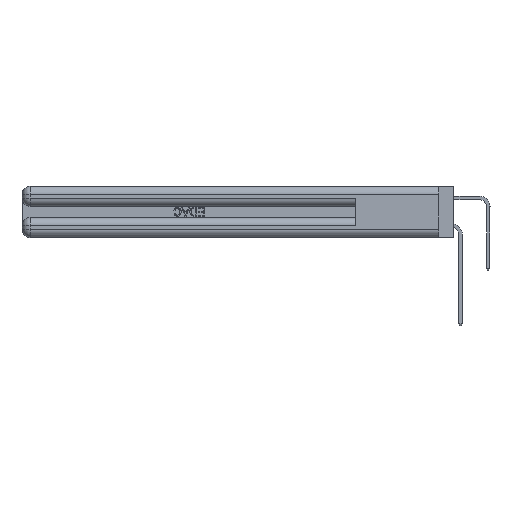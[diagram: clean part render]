
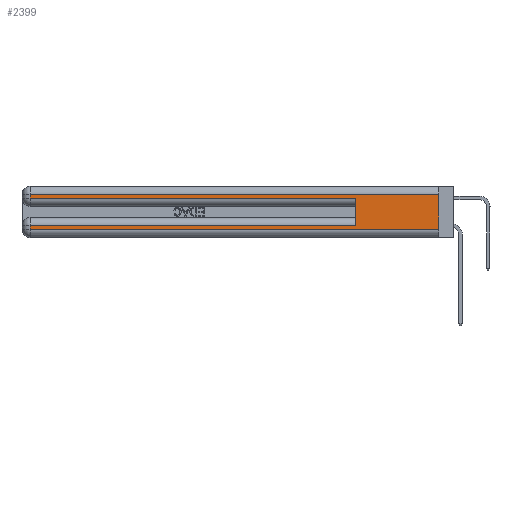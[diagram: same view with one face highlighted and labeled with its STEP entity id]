
A CAD part, left-side view. The second image highlights one B-rep face of the part: STEP entity #2399.
In plain terms, the highlighted planar face has unit normal (-1, 0, 0).
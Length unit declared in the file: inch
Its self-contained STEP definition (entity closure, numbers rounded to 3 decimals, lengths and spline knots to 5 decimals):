
#1094 = DIRECTION ( 'NONE',  ( 0., -1., 0. ) ) ;
#1205 = EDGE_CURVE ( 'NONE', #32645, #39011, #16985, .T. ) ;
#1219 = VECTOR ( 'NONE', #8162, 39.37008 ) ;
#2399 = ADVANCED_FACE ( 'NONE', ( #38661 ), #8370, .F. ) ;
#2451 = LINE ( 'NONE', #16035, #1219 ) ;
#2723 = VERTEX_POINT ( 'NONE', #14135 ) ;
#2846 = CARTESIAN_POINT ( 'NONE',  ( 0., 2.94, 0.085 ) ) ;
#3586 = LINE ( 'NONE', #7741, #32290 ) ;
#4106 = ORIENTED_EDGE ( 'NONE', *, *, #9121, .T. ) ;
#4197 = CARTESIAN_POINT ( 'NONE',  ( 0., 2.94, 0.31 ) ) ;
#4826 = EDGE_CURVE ( 'NONE', #7121, #41956, #14136, .T. ) ;
#6564 = VECTOR ( 'NONE', #32512, 39.37008 ) ;
#7035 = LINE ( 'NONE', #35326, #14987 ) ;
#7121 = VERTEX_POINT ( 'NONE', #18019 ) ;
#7741 = CARTESIAN_POINT ( 'NONE',  ( 0., 0., 0.085 ) ) ;
#8162 = DIRECTION ( 'NONE',  ( 0., 0., 1. ) ) ;
#8217 = CARTESIAN_POINT ( 'NONE',  ( 0., 2.94, 0.37 ) ) ;
#8275 = ORIENTED_EDGE ( 'NONE', *, *, #17994, .T. ) ;
#8370 = PLANE ( 'NONE',  #22310 ) ;
#8657 = ORIENTED_EDGE ( 'NONE', *, *, #4826, .T. ) ;
#9121 = EDGE_CURVE ( 'NONE', #40949, #32645, #15462, .T. ) ;
#10954 = VECTOR ( 'NONE', #39258, 39.37008 ) ;
#12093 = CARTESIAN_POINT ( 'NONE',  ( 0., 0., 0.31 ) ) ;
#12893 = VECTOR ( 'NONE', #1094, 39.37008 ) ;
#14135 = CARTESIAN_POINT ( 'NONE',  ( 0., 0.6, 0.085 ) ) ;
#14136 = LINE ( 'NONE', #47698, #12893 ) ;
#14987 = VECTOR ( 'NONE', #39172, 39.37008 ) ;
#15432 = CARTESIAN_POINT ( 'NONE',  ( 0., 0., 0.06 ) ) ;
#15462 = LINE ( 'NONE', #8217, #42700 ) ;
#15666 = VERTEX_POINT ( 'NONE', #43727 ) ;
#16035 = CARTESIAN_POINT ( 'NONE',  ( 0., 0.6, 0.145 ) ) ;
#16252 = EDGE_LOOP ( 'NONE', ( #17455, #21763, #4106, #31631, #39479, #26486, #8275, #8657 ) ) ;
#16850 = CARTESIAN_POINT ( 'NONE',  ( 0., 2.94, 0.37 ) ) ;
#16985 = LINE ( 'NONE', #28604, #6564 ) ;
#17455 = ORIENTED_EDGE ( 'NONE', *, *, #45532, .F. ) ;
#17994 = EDGE_CURVE ( 'NONE', #44722, #7121, #19806, .T. ) ;
#18019 = CARTESIAN_POINT ( 'NONE',  ( 0., 2.94, 0.06 ) ) ;
#18576 = VECTOR ( 'NONE', #43878, 39.37008 ) ;
#19806 = LINE ( 'NONE', #16850, #18576 ) ;
#20209 = CARTESIAN_POINT ( 'NONE',  ( 0., 0., 0.37 ) ) ;
#21763 = ORIENTED_EDGE ( 'NONE', *, *, #32632, .T. ) ;
#22310 = AXIS2_PLACEMENT_3D ( 'NONE', #20209, #47226, #24056 ) ;
#24056 = DIRECTION ( 'NONE',  ( 0., 0., -1. ) ) ;
#26486 = ORIENTED_EDGE ( 'NONE', *, *, #33580, .T. ) ;
#28604 = CARTESIAN_POINT ( 'NONE',  ( 0., 0., 0.285 ) ) ;
#31631 = ORIENTED_EDGE ( 'NONE', *, *, #1205, .T. ) ;
#32290 = VECTOR ( 'NONE', #42666, 39.37008 ) ;
#32512 = DIRECTION ( 'NONE',  ( 0., -1., 0. ) ) ;
#32632 = EDGE_CURVE ( 'NONE', #15666, #40949, #41899, .T. ) ;
#32645 = VERTEX_POINT ( 'NONE', #47051 ) ;
#33580 = EDGE_CURVE ( 'NONE', #2723, #44722, #3586, .T. ) ;
#35326 = CARTESIAN_POINT ( 'NONE',  ( 0., 0., 0.37 ) ) ;
#38661 = FACE_OUTER_BOUND ( 'NONE', #16252, .T. ) ;
#38713 = EDGE_CURVE ( 'NONE', #2723, #39011, #2451, .T. ) ;
#39011 = VERTEX_POINT ( 'NONE', #46671 ) ;
#39172 = DIRECTION ( 'NONE',  ( 0., 0., -1. ) ) ;
#39258 = DIRECTION ( 'NONE',  ( 0., 1., 0. ) ) ;
#39276 = DIRECTION ( 'NONE',  ( 0., 0., -1. ) ) ;
#39479 = ORIENTED_EDGE ( 'NONE', *, *, #38713, .F. ) ;
#40949 = VERTEX_POINT ( 'NONE', #4197 ) ;
#41899 = LINE ( 'NONE', #12093, #10954 ) ;
#41956 = VERTEX_POINT ( 'NONE', #15432 ) ;
#42666 = DIRECTION ( 'NONE',  ( 0., 1., 0. ) ) ;
#42700 = VECTOR ( 'NONE', #39276, 39.37008 ) ;
#43727 = CARTESIAN_POINT ( 'NONE',  ( 0., 0., 0.31 ) ) ;
#43878 = DIRECTION ( 'NONE',  ( 0., 0., -1. ) ) ;
#44722 = VERTEX_POINT ( 'NONE', #2846 ) ;
#45532 = EDGE_CURVE ( 'NONE', #15666, #41956, #7035, .T. ) ;
#46671 = CARTESIAN_POINT ( 'NONE',  ( 0., 0.6, 0.285 ) ) ;
#47051 = CARTESIAN_POINT ( 'NONE',  ( 0., 2.94, 0.285 ) ) ;
#47226 = DIRECTION ( 'NONE',  ( 1., 0., 0. ) ) ;
#47698 = CARTESIAN_POINT ( 'NONE',  ( 0., 0., 0.06 ) ) ;
